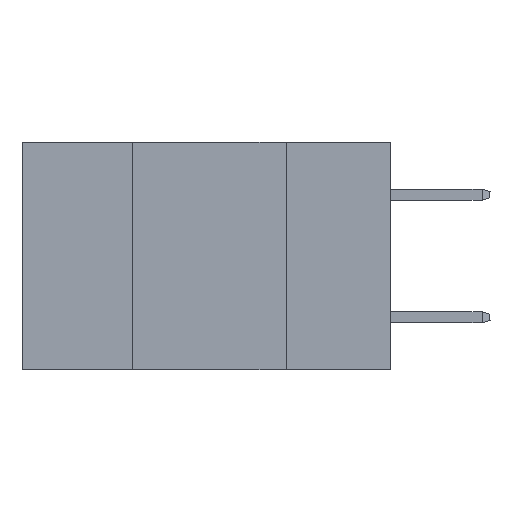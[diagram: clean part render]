
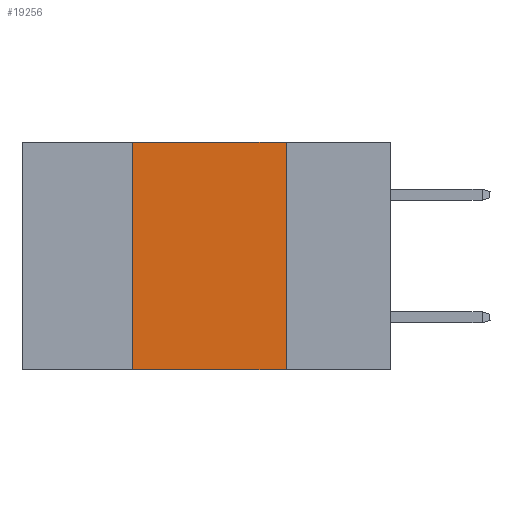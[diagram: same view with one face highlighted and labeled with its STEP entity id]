
A CAD part, left-side view. The second image highlights one B-rep face of the part: STEP entity #19256.
In plain terms, the highlighted planar face has unit normal (-1, 0, 0).
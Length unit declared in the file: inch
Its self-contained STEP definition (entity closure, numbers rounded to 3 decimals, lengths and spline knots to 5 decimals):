
#117 = CARTESIAN_POINT ( 'NONE',  ( 0., 0.17, -0.37 ) ) ;
#480 = CARTESIAN_POINT ( 'NONE',  ( 0., 0.6, 0. ) ) ;
#1332 = DIRECTION ( 'NONE',  ( 0., 0., 1. ) ) ;
#1703 = LINE ( 'NONE', #20188, #5719 ) ;
#2032 = LINE ( 'NONE', #14935, #18539 ) ;
#2212 = DIRECTION ( 'NONE',  ( 0., -1., 0. ) ) ;
#3797 = VERTEX_POINT ( 'NONE', #19272 ) ;
#4037 = FACE_OUTER_BOUND ( 'NONE', #9184, .T. ) ;
#4709 = CARTESIAN_POINT ( 'NONE',  ( 0., 0.6, 0. ) ) ;
#5072 = ORIENTED_EDGE ( 'NONE', *, *, #10734, .F. ) ;
#5719 = VECTOR ( 'NONE', #8939, 39.37008 ) ;
#5847 = LINE ( 'NONE', #480, #9803 ) ;
#6006 = CARTESIAN_POINT ( 'NONE',  ( 0., 0.17, 0. ) ) ;
#6679 = ORIENTED_EDGE ( 'NONE', *, *, #13846, .F. ) ;
#8130 = EDGE_CURVE ( 'NONE', #14449, #11623, #5847, .T. ) ;
#8137 = DIRECTION ( 'NONE',  ( 1., 0., 0. ) ) ;
#8148 = CARTESIAN_POINT ( 'NONE',  ( 0., 0.42, 0. ) ) ;
#8939 = DIRECTION ( 'NONE',  ( 0., 0., -1. ) ) ;
#9184 = EDGE_LOOP ( 'NONE', ( #5072, #14374, #6679, #16412 ) ) ;
#9803 = VECTOR ( 'NONE', #2212, 39.37008 ) ;
#10011 = AXIS2_PLACEMENT_3D ( 'NONE', #4709, #8137, #19421 ) ;
#10637 = VERTEX_POINT ( 'NONE', #117 ) ;
#10734 = EDGE_CURVE ( 'NONE', #11623, #10637, #1703, .T. ) ;
#11238 = CARTESIAN_POINT ( 'NONE',  ( 0., 0.42, 0. ) ) ;
#11623 = VERTEX_POINT ( 'NONE', #6006 ) ;
#13846 = EDGE_CURVE ( 'NONE', #3797, #14449, #15641, .T. ) ;
#14374 = ORIENTED_EDGE ( 'NONE', *, *, #8130, .F. ) ;
#14449 = VERTEX_POINT ( 'NONE', #11238 ) ;
#14935 = CARTESIAN_POINT ( 'NONE',  ( 0., 0.6, -0.37 ) ) ;
#15641 = LINE ( 'NONE', #8148, #19878 ) ;
#15903 = EDGE_CURVE ( 'NONE', #3797, #10637, #2032, .T. ) ;
#16412 = ORIENTED_EDGE ( 'NONE', *, *, #15903, .T. ) ;
#17822 = PLANE ( 'NONE',  #10011 ) ;
#18539 = VECTOR ( 'NONE', #19766, 39.37008 ) ;
#19256 = ADVANCED_FACE ( 'NONE', ( #4037 ), #17822, .F. ) ;
#19272 = CARTESIAN_POINT ( 'NONE',  ( 0., 0.42, -0.37 ) ) ;
#19421 = DIRECTION ( 'NONE',  ( 0., 0., -1. ) ) ;
#19766 = DIRECTION ( 'NONE',  ( 0., -1., 0. ) ) ;
#19878 = VECTOR ( 'NONE', #1332, 39.37008 ) ;
#20188 = CARTESIAN_POINT ( 'NONE',  ( 0., 0.17, 0. ) ) ;
